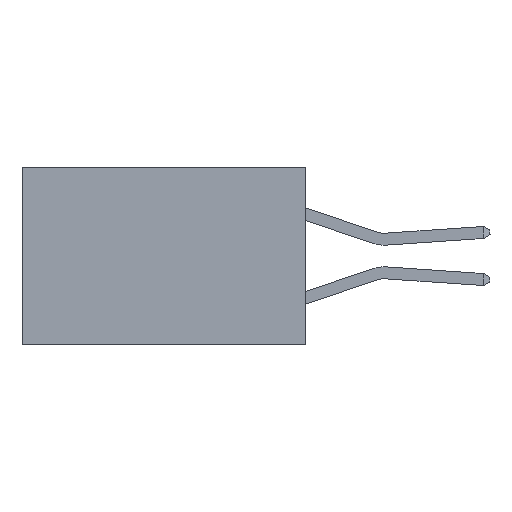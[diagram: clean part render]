
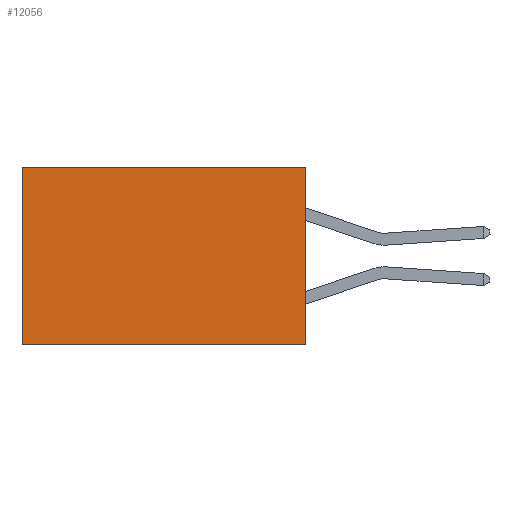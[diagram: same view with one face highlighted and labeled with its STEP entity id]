
A CAD part, left-side view. The second image highlights one B-rep face of the part: STEP entity #12056.
In plain terms, the highlighted planar face has unit normal (-1, 0, 0).
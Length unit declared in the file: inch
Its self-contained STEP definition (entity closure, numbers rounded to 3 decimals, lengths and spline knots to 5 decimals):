
#1614 = VERTEX_POINT ( 'NONE', #7821 ) ;
#1750 = EDGE_CURVE ( 'NONE', #11130, #12545, #16313, .T. ) ;
#2334 = DIRECTION ( 'NONE',  ( 0., 1., 0. ) ) ;
#2478 = VECTOR ( 'NONE', #13365, 39.37008 ) ;
#4212 = LINE ( 'NONE', #16328, #11567 ) ;
#6214 = CARTESIAN_POINT ( 'NONE',  ( 0.277, 0., -0.37 ) ) ;
#6517 = DIRECTION ( 'NONE',  ( 0., 0., -1. ) ) ;
#7251 = EDGE_CURVE ( 'NONE', #1614, #9213, #4212, .T. ) ;
#7686 = ORIENTED_EDGE ( 'NONE', *, *, #16380, .F. ) ;
#7821 = CARTESIAN_POINT ( 'NONE',  ( 0.277, 0., 0. ) ) ;
#8113 = DIRECTION ( 'NONE',  ( 0., 0., -1. ) ) ;
#9213 = VERTEX_POINT ( 'NONE', #9403 ) ;
#9403 = CARTESIAN_POINT ( 'NONE',  ( 0.277, 0.59, 0. ) ) ;
#10090 = VECTOR ( 'NONE', #6517, 39.37008 ) ;
#10594 = CARTESIAN_POINT ( 'NONE',  ( 0.277, 0.59, -0.37 ) ) ;
#11130 = VERTEX_POINT ( 'NONE', #12655 ) ;
#11523 = AXIS2_PLACEMENT_3D ( 'NONE', #15309, #16633, #8113 ) ;
#11567 = VECTOR ( 'NONE', #16248, 39.37008 ) ;
#12056 = ADVANCED_FACE ( 'NONE', ( #12674 ), #13922, .F. ) ;
#12165 = VECTOR ( 'NONE', #2334, 39.37008 ) ;
#12545 = VERTEX_POINT ( 'NONE', #10594 ) ;
#12655 = CARTESIAN_POINT ( 'NONE',  ( 0.277, 0., -0.37 ) ) ;
#12674 = FACE_OUTER_BOUND ( 'NONE', #15218, .T. ) ;
#13300 = CARTESIAN_POINT ( 'NONE',  ( 0.277, 0.59, -0.37 ) ) ;
#13365 = DIRECTION ( 'NONE',  ( 0., 0., -1. ) ) ;
#13922 = PLANE ( 'NONE',  #11523 ) ;
#14178 = LINE ( 'NONE', #13300, #2478 ) ;
#14307 = ORIENTED_EDGE ( 'NONE', *, *, #7251, .T. ) ;
#15165 = CARTESIAN_POINT ( 'NONE',  ( 0.277, 0., -0.37 ) ) ;
#15218 = EDGE_LOOP ( 'NONE', ( #16793, #16624, #7686, #14307 ) ) ;
#15309 = CARTESIAN_POINT ( 'NONE',  ( 0.277, 0., -0.37 ) ) ;
#16180 = EDGE_CURVE ( 'NONE', #9213, #12545, #14178, .T. ) ;
#16248 = DIRECTION ( 'NONE',  ( 0., 1., 0. ) ) ;
#16313 = LINE ( 'NONE', #6214, #12165 ) ;
#16328 = CARTESIAN_POINT ( 'NONE',  ( 0.277, 0., 0. ) ) ;
#16380 = EDGE_CURVE ( 'NONE', #1614, #11130, #17107, .T. ) ;
#16624 = ORIENTED_EDGE ( 'NONE', *, *, #1750, .F. ) ;
#16633 = DIRECTION ( 'NONE',  ( 1., 0., 0. ) ) ;
#16793 = ORIENTED_EDGE ( 'NONE', *, *, #16180, .T. ) ;
#17107 = LINE ( 'NONE', #15165, #10090 ) ;
